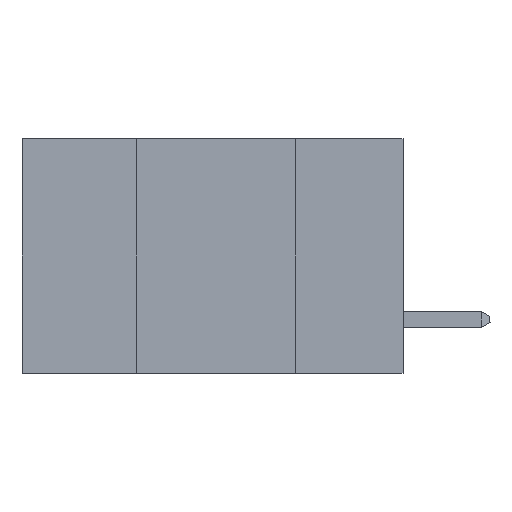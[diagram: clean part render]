
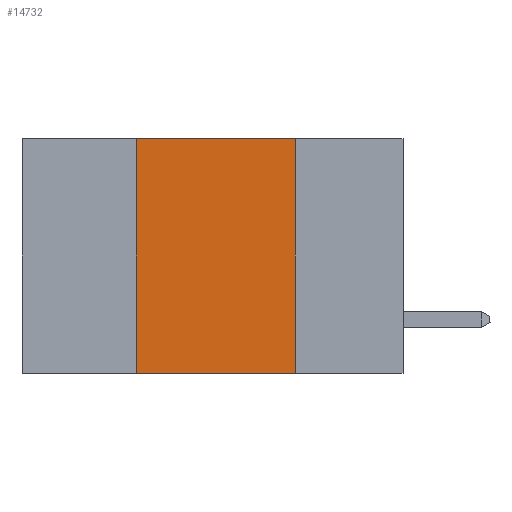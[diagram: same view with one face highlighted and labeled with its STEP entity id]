
A CAD part, left-side view. The second image highlights one B-rep face of the part: STEP entity #14732.
In plain terms, the highlighted planar face has unit normal (-1, 0, 0).
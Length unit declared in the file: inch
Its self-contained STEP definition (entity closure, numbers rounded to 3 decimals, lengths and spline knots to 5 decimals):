
#5135 = AXIS2_PLACEMENT_3D ( 'NONE', #28205, #35131, #11870 ) ;
#5749 = ORIENTED_EDGE ( 'NONE', *, *, #12338, .F. ) ;
#5813 = DIRECTION ( 'NONE',  ( 0., 0., 1. ) ) ;
#7692 = LINE ( 'NONE', #24402, #35579 ) ;
#11702 = VERTEX_POINT ( 'NONE', #18793 ) ;
#11870 = DIRECTION ( 'NONE',  ( 0., 0., -1. ) ) ;
#12338 = EDGE_CURVE ( 'NONE', #24662, #47021, #30875, .T. ) ;
#12918 = LINE ( 'NONE', #21738, #31158 ) ;
#14022 = EDGE_LOOP ( 'NONE', ( #30802, #5749, #49246, #35659 ) ) ;
#14732 = ADVANCED_FACE ( 'NONE', ( #15463 ), #32082, .F. ) ;
#15463 = FACE_OUTER_BOUND ( 'NONE', #14022, .T. ) ;
#15872 = CARTESIAN_POINT ( 'NONE',  ( 0., 0.6, 0. ) ) ;
#18668 = CARTESIAN_POINT ( 'NONE',  ( 0., 0.42, 0. ) ) ;
#18793 = CARTESIAN_POINT ( 'NONE',  ( 0., 0.42, -0.37 ) ) ;
#21738 = CARTESIAN_POINT ( 'NONE',  ( 0., 0.42, 0. ) ) ;
#24402 = CARTESIAN_POINT ( 'NONE',  ( 0., 0.6, -0.37 ) ) ;
#24662 = VERTEX_POINT ( 'NONE', #18668 ) ;
#27074 = EDGE_CURVE ( 'NONE', #11702, #41946, #7692, .T. ) ;
#27665 = DIRECTION ( 'NONE',  ( 0., 0., -1. ) ) ;
#27784 = LINE ( 'NONE', #35774, #46041 ) ;
#28205 = CARTESIAN_POINT ( 'NONE',  ( 0., 0.6, 0. ) ) ;
#30430 = CARTESIAN_POINT ( 'NONE',  ( 0., 0.17, -0.37 ) ) ;
#30802 = ORIENTED_EDGE ( 'NONE', *, *, #40589, .F. ) ;
#30875 = LINE ( 'NONE', #15872, #33285 ) ;
#31158 = VECTOR ( 'NONE', #5813, 39.37008 ) ;
#31587 = CARTESIAN_POINT ( 'NONE',  ( 0., 0.17, 0. ) ) ;
#32082 = PLANE ( 'NONE',  #5135 ) ;
#33285 = VECTOR ( 'NONE', #35411, 39.37008 ) ;
#35131 = DIRECTION ( 'NONE',  ( 1., 0., 0. ) ) ;
#35411 = DIRECTION ( 'NONE',  ( 0., -1., 0. ) ) ;
#35579 = VECTOR ( 'NONE', #48194, 39.37008 ) ;
#35659 = ORIENTED_EDGE ( 'NONE', *, *, #27074, .T. ) ;
#35774 = CARTESIAN_POINT ( 'NONE',  ( 0., 0.17, 0. ) ) ;
#40589 = EDGE_CURVE ( 'NONE', #47021, #41946, #27784, .T. ) ;
#41946 = VERTEX_POINT ( 'NONE', #30430 ) ;
#46041 = VECTOR ( 'NONE', #27665, 39.37008 ) ;
#47021 = VERTEX_POINT ( 'NONE', #31587 ) ;
#47754 = EDGE_CURVE ( 'NONE', #11702, #24662, #12918, .T. ) ;
#48194 = DIRECTION ( 'NONE',  ( 0., -1., 0. ) ) ;
#49246 = ORIENTED_EDGE ( 'NONE', *, *, #47754, .F. ) ;
